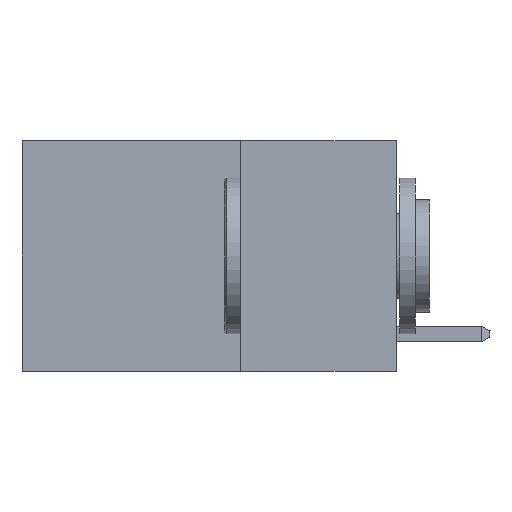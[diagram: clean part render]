
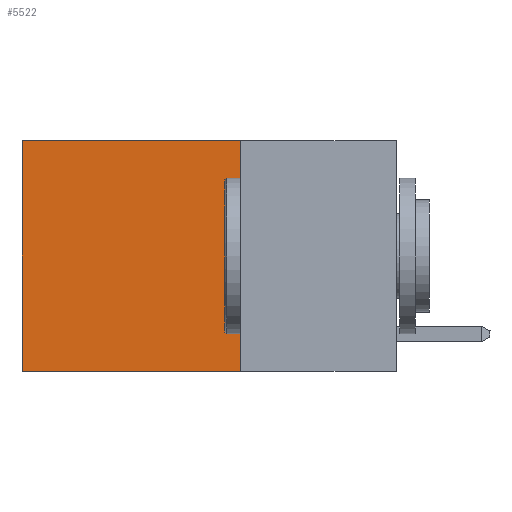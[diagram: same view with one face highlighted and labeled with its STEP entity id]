
A CAD part, left-side view. The second image highlights one B-rep face of the part: STEP entity #5522.
In plain terms, the highlighted planar face has unit normal (-1, 0, 0).
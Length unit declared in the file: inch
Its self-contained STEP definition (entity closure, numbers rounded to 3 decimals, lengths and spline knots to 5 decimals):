
#120 = AXIS2_PLACEMENT_3D ( 'NONE', #5842, #899, #5877 ) ;
#300 = ORIENTED_EDGE ( 'NONE', *, *, #7077, .T. ) ;
#633 = CARTESIAN_POINT ( 'NONE',  ( 0.2625, 0.6, 0. ) ) ;
#650 = VECTOR ( 'NONE', #4434, 39.37008 ) ;
#876 = EDGE_CURVE ( 'NONE', #7804, #947, #2796, .T. ) ;
#899 = DIRECTION ( 'NONE',  ( 1., 0., 0. ) ) ;
#947 = VERTEX_POINT ( 'NONE', #7327 ) ;
#1826 = PLANE ( 'NONE',  #120 ) ;
#2256 = DIRECTION ( 'NONE',  ( 0., 0., -1. ) ) ;
#2325 = CARTESIAN_POINT ( 'NONE',  ( 0.2625, 0.25, 0. ) ) ;
#2796 = LINE ( 'NONE', #9592, #3070 ) ;
#3070 = VECTOR ( 'NONE', #2256, 39.37008 ) ;
#3414 = LINE ( 'NONE', #2325, #5958 ) ;
#3760 = DIRECTION ( 'NONE',  ( 0., 0., -1. ) ) ;
#3973 = ORIENTED_EDGE ( 'NONE', *, *, #876, .T. ) ;
#4209 = VECTOR ( 'NONE', #3760, 39.37008 ) ;
#4434 = DIRECTION ( 'NONE',  ( 0., 1., 0. ) ) ;
#4778 = DIRECTION ( 'NONE',  ( 0., 1., 0. ) ) ;
#4924 = ORIENTED_EDGE ( 'NONE', *, *, #8574, .F. ) ;
#5522 = ADVANCED_FACE ( 'NONE', ( #8097 ), #1826, .F. ) ;
#5723 = EDGE_CURVE ( 'NONE', #10006, #947, #8351, .T. ) ;
#5842 = CARTESIAN_POINT ( 'NONE',  ( 0.2625, 0.25, 0. ) ) ;
#5858 = EDGE_LOOP ( 'NONE', ( #3973, #9205, #4924, #300 ) ) ;
#5877 = DIRECTION ( 'NONE',  ( 0., 0., -1. ) ) ;
#5958 = VECTOR ( 'NONE', #4778, 39.37008 ) ;
#6073 = VERTEX_POINT ( 'NONE', #7166 ) ;
#6373 = LINE ( 'NONE', #7010, #4209 ) ;
#7010 = CARTESIAN_POINT ( 'NONE',  ( 0.2625, 0.25, 0. ) ) ;
#7077 = EDGE_CURVE ( 'NONE', #6073, #7804, #3414, .T. ) ;
#7166 = CARTESIAN_POINT ( 'NONE',  ( 0.2625, 0.25, 0. ) ) ;
#7327 = CARTESIAN_POINT ( 'NONE',  ( 0.2625, 0.6, -0.37 ) ) ;
#7804 = VERTEX_POINT ( 'NONE', #633 ) ;
#8097 = FACE_OUTER_BOUND ( 'NONE', #5858, .T. ) ;
#8351 = LINE ( 'NONE', #10183, #650 ) ;
#8574 = EDGE_CURVE ( 'NONE', #6073, #10006, #6373, .T. ) ;
#9205 = ORIENTED_EDGE ( 'NONE', *, *, #5723, .F. ) ;
#9274 = CARTESIAN_POINT ( 'NONE',  ( 0.2625, 0.25, -0.37 ) ) ;
#9592 = CARTESIAN_POINT ( 'NONE',  ( 0.2625, 0.6, 0. ) ) ;
#10006 = VERTEX_POINT ( 'NONE', #9274 ) ;
#10183 = CARTESIAN_POINT ( 'NONE',  ( 0.2625, 0.25, -0.37 ) ) ;
